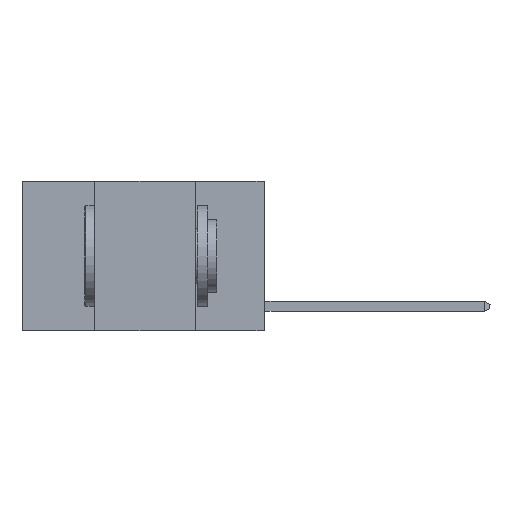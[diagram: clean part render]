
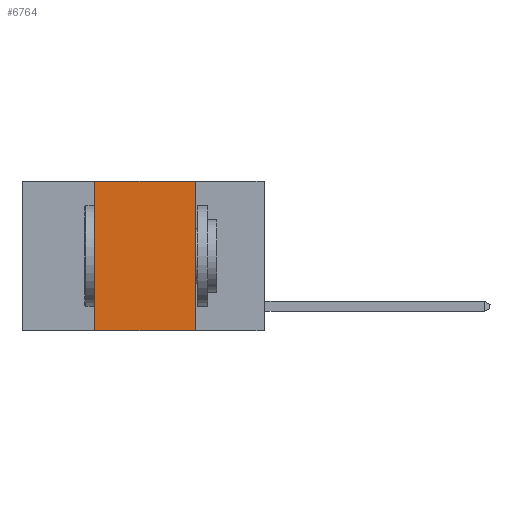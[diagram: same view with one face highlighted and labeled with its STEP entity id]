
A CAD part, left-side view. The second image highlights one B-rep face of the part: STEP entity #6764.
In plain terms, the highlighted planar face has unit normal (-1, 0, 0).
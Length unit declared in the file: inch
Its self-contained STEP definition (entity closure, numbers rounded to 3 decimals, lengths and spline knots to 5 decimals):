
#724 = CARTESIAN_POINT ( 'NONE',  ( 0., 0.6, -0.37 ) ) ;
#1107 = ORIENTED_EDGE ( 'NONE', *, *, #8086, .F. ) ;
#1247 = FACE_OUTER_BOUND ( 'NONE', #3983, .T. ) ;
#1390 = LINE ( 'NONE', #11618, #5468 ) ;
#1674 = VERTEX_POINT ( 'NONE', #13084 ) ;
#2069 = DIRECTION ( 'NONE',  ( 1., 0., 0. ) ) ;
#2120 = DIRECTION ( 'NONE',  ( 0., -1., 0. ) ) ;
#2153 = CARTESIAN_POINT ( 'NONE',  ( 0., 0.6, 0. ) ) ;
#2707 = EDGE_CURVE ( 'NONE', #4868, #1674, #8707, .T. ) ;
#3192 = CARTESIAN_POINT ( 'NONE',  ( 0., 0.17, 0. ) ) ;
#3899 = EDGE_CURVE ( 'NONE', #1674, #15835, #9940, .T. ) ;
#3983 = EDGE_LOOP ( 'NONE', ( #1107, #10205, #15754, #8746 ) ) ;
#4868 = VERTEX_POINT ( 'NONE', #9490 ) ;
#5468 = VECTOR ( 'NONE', #16927, 39.37008 ) ;
#6165 = PLANE ( 'NONE',  #13611 ) ;
#6764 = ADVANCED_FACE ( 'NONE', ( #1247 ), #6165, .F. ) ;
#7866 = VECTOR ( 'NONE', #13793, 39.37008 ) ;
#8086 = EDGE_CURVE ( 'NONE', #15835, #16213, #1390, .T. ) ;
#8163 = CARTESIAN_POINT ( 'NONE',  ( 0., 0.17, -0.37 ) ) ;
#8707 = LINE ( 'NONE', #14137, #7866 ) ;
#8746 = ORIENTED_EDGE ( 'NONE', *, *, #12554, .T. ) ;
#9490 = CARTESIAN_POINT ( 'NONE',  ( 0., 0.42, -0.37 ) ) ;
#9940 = LINE ( 'NONE', #2153, #16664 ) ;
#10205 = ORIENTED_EDGE ( 'NONE', *, *, #3899, .F. ) ;
#10275 = CARTESIAN_POINT ( 'NONE',  ( 0., 0.6, 0. ) ) ;
#11618 = CARTESIAN_POINT ( 'NONE',  ( 0., 0.17, 0. ) ) ;
#11655 = DIRECTION ( 'NONE',  ( 0., 0., -1. ) ) ;
#12554 = EDGE_CURVE ( 'NONE', #4868, #16213, #16320, .T. ) ;
#12774 = VECTOR ( 'NONE', #2120, 39.37008 ) ;
#13072 = DIRECTION ( 'NONE',  ( 0., -1., 0. ) ) ;
#13084 = CARTESIAN_POINT ( 'NONE',  ( 0., 0.42, 0. ) ) ;
#13611 = AXIS2_PLACEMENT_3D ( 'NONE', #10275, #2069, #11655 ) ;
#13793 = DIRECTION ( 'NONE',  ( 0., 0., 1. ) ) ;
#14137 = CARTESIAN_POINT ( 'NONE',  ( 0., 0.42, 0. ) ) ;
#15754 = ORIENTED_EDGE ( 'NONE', *, *, #2707, .F. ) ;
#15835 = VERTEX_POINT ( 'NONE', #3192 ) ;
#16213 = VERTEX_POINT ( 'NONE', #8163 ) ;
#16320 = LINE ( 'NONE', #724, #12774 ) ;
#16664 = VECTOR ( 'NONE', #13072, 39.37008 ) ;
#16927 = DIRECTION ( 'NONE',  ( 0., 0., -1. ) ) ;
